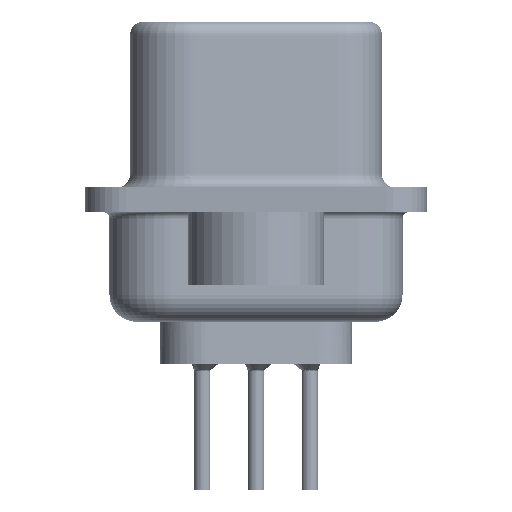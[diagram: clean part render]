
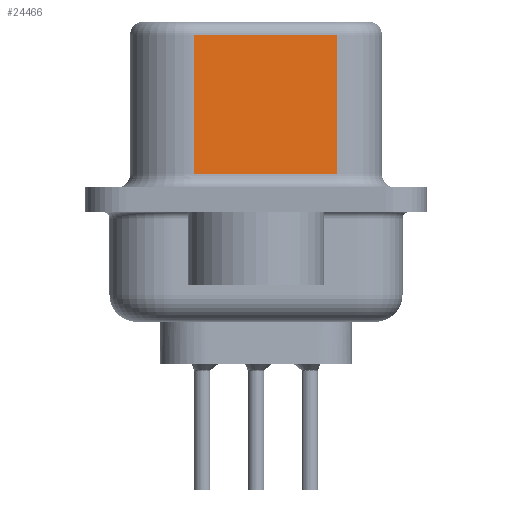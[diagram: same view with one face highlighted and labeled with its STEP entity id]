
A CAD part, left-side view. The second image highlights one B-rep face of the part: STEP entity #24466.
In plain terms, the highlighted planar face has unit normal (-0.985, -0.174, 0).
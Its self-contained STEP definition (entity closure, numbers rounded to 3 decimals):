
#16 = FACE_OUTER_BOUND ( 'NONE', #26126, .T. ) ;
#2841 = DIRECTION ( 'NONE',  ( 0., 0., -1. ) ) ;
#2994 = DIRECTION ( 'NONE',  ( -0.174, 0.985, 0. ) ) ;
#4146 = VERTEX_POINT ( 'NONE', #20988 ) ;
#4774 = ORIENTED_EDGE ( 'NONE', *, *, #20921, .T. ) ;
#5057 = ORIENTED_EDGE ( 'NONE', *, *, #29107, .T. ) ;
#5273 = PLANE ( 'NONE',  #32977 ) ;
#5449 = ORIENTED_EDGE ( 'NONE', *, *, #26668, .F. ) ;
#12350 = VERTEX_POINT ( 'NONE', #20653 ) ;
#13508 = VECTOR ( 'NONE', #22271, 1000. ) ;
#14376 = ORIENTED_EDGE ( 'NONE', *, *, #21361, .T. ) ;
#15574 = DIRECTION ( 'NONE',  ( 0.174, -0.985, 0. ) ) ;
#17289 = CARTESIAN_POINT ( 'NONE',  ( 3.62, 2.293, 6.07 ) ) ;
#17368 = CARTESIAN_POINT ( 'NONE',  ( 4.551, -2.987, 6.57 ) ) ;
#18259 = CARTESIAN_POINT ( 'NONE',  ( 3.62, 2.293, 6.57 ) ) ;
#18644 = VERTEX_POINT ( 'NONE', #22782 ) ;
#20100 = VECTOR ( 'NONE', #2841, 1000. ) ;
#20381 = VECTOR ( 'NONE', #15574, 1000. ) ;
#20653 = CARTESIAN_POINT ( 'NONE',  ( 4.551, -2.987, 0.95 ) ) ;
#20789 = LINE ( 'NONE', #18259, #20100 ) ;
#20921 = EDGE_CURVE ( 'NONE', #18644, #12350, #28094, .T. ) ;
#20988 = CARTESIAN_POINT ( 'NONE',  ( 4.551, -2.987, 6.07 ) ) ;
#21272 = CARTESIAN_POINT ( 'NONE',  ( 4.551, -2.987, 6.07 ) ) ;
#21361 = EDGE_CURVE ( 'NONE', #4146, #27081, #29046, .T. ) ;
#22271 = DIRECTION ( 'NONE',  ( 0., 0., -1. ) ) ;
#22782 = CARTESIAN_POINT ( 'NONE',  ( 3.62, 2.293, 0.95 ) ) ;
#24466 = ADVANCED_FACE ( 'NONE', ( #16 ), #5273, .F. ) ;
#25153 = LINE ( 'NONE', #17368, #13508 ) ;
#26126 = EDGE_LOOP ( 'NONE', ( #5449, #14376, #5057, #4774 ) ) ;
#26668 = EDGE_CURVE ( 'NONE', #4146, #12350, #25153, .T. ) ;
#27081 = VERTEX_POINT ( 'NONE', #17289 ) ;
#27397 = VECTOR ( 'NONE', #2994, 1000. ) ;
#28094 = LINE ( 'NONE', #30463, #20381 ) ;
#28774 = CARTESIAN_POINT ( 'NONE',  ( 4.551, -2.987, 6.57 ) ) ;
#29046 = LINE ( 'NONE', #21272, #27397 ) ;
#29107 = EDGE_CURVE ( 'NONE', #27081, #18644, #20789, .T. ) ;
#29275 = DIRECTION ( 'NONE',  ( -0.174, 0.985, 0. ) ) ;
#30463 = CARTESIAN_POINT ( 'NONE',  ( 4.551, -2.987, 0.95 ) ) ;
#31814 = DIRECTION ( 'NONE',  ( 0.985, 0.174, 0. ) ) ;
#32977 = AXIS2_PLACEMENT_3D ( 'NONE', #28774, #31814, #29275 ) ;
